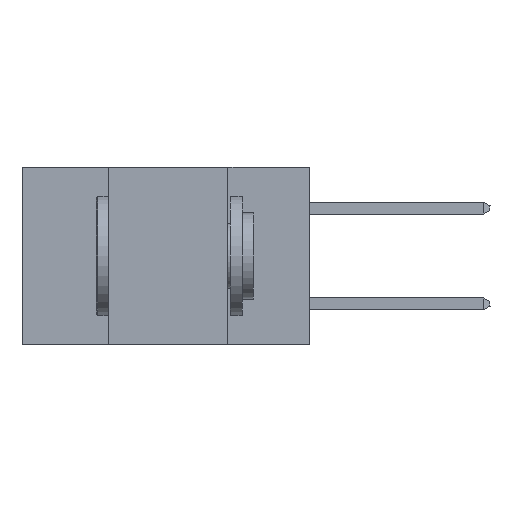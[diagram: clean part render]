
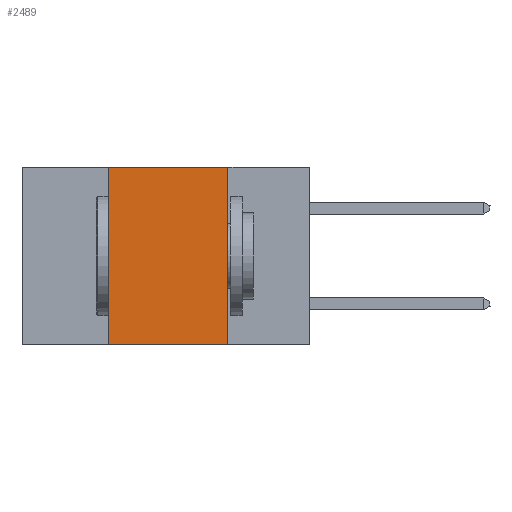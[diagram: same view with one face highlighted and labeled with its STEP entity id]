
A CAD part, left-side view. The second image highlights one B-rep face of the part: STEP entity #2489.
In plain terms, the highlighted planar face has unit normal (-1, 0, 0).
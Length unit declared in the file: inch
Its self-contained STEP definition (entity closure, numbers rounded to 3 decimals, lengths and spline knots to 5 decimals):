
#220 = EDGE_CURVE ( 'NONE', #19680, #14935, #5817, .T. ) ;
#1143 = DIRECTION ( 'NONE',  ( 0., -1., 0. ) ) ;
#2178 = ORIENTED_EDGE ( 'NONE', *, *, #21075, .F. ) ;
#2489 = ADVANCED_FACE ( 'NONE', ( #11546 ), #8200, .F. ) ;
#2505 = CARTESIAN_POINT ( 'NONE',  ( 0., 0.6, 0. ) ) ;
#5447 = CARTESIAN_POINT ( 'NONE',  ( 0., 0.17, -0.37 ) ) ;
#5817 = LINE ( 'NONE', #8719, #15392 ) ;
#6042 = CARTESIAN_POINT ( 'NONE',  ( 0., 0.17, 0. ) ) ;
#6804 = EDGE_LOOP ( 'NONE', ( #15259, #20883, #2178, #8246 ) ) ;
#8001 = EDGE_CURVE ( 'NONE', #12782, #14935, #11087, .T. ) ;
#8118 = DIRECTION ( 'NONE',  ( 1., 0., 0. ) ) ;
#8200 = PLANE ( 'NONE',  #21319 ) ;
#8246 = ORIENTED_EDGE ( 'NONE', *, *, #220, .T. ) ;
#8443 = LINE ( 'NONE', #20289, #19473 ) ;
#8719 = CARTESIAN_POINT ( 'NONE',  ( 0., 0.6, -0.37 ) ) ;
#10296 = DIRECTION ( 'NONE',  ( 0., 0., 1. ) ) ;
#11087 = LINE ( 'NONE', #6042, #20639 ) ;
#11336 = CARTESIAN_POINT ( 'NONE',  ( 0., 0.42, -0.37 ) ) ;
#11546 = FACE_OUTER_BOUND ( 'NONE', #6804, .T. ) ;
#11783 = CARTESIAN_POINT ( 'NONE',  ( 0., 0.42, 0. ) ) ;
#11793 = DIRECTION ( 'NONE',  ( 0., 0., -1. ) ) ;
#11821 = DIRECTION ( 'NONE',  ( 0., 0., -1. ) ) ;
#12782 = VERTEX_POINT ( 'NONE', #19895 ) ;
#13041 = DIRECTION ( 'NONE',  ( 0., -1., 0. ) ) ;
#13751 = LINE ( 'NONE', #16105, #19305 ) ;
#14935 = VERTEX_POINT ( 'NONE', #5447 ) ;
#15259 = ORIENTED_EDGE ( 'NONE', *, *, #8001, .F. ) ;
#15392 = VECTOR ( 'NONE', #1143, 39.37008 ) ;
#16105 = CARTESIAN_POINT ( 'NONE',  ( 0., 0.42, 0. ) ) ;
#19305 = VECTOR ( 'NONE', #10296, 39.37008 ) ;
#19392 = VERTEX_POINT ( 'NONE', #11783 ) ;
#19473 = VECTOR ( 'NONE', #13041, 39.37008 ) ;
#19680 = VERTEX_POINT ( 'NONE', #11336 ) ;
#19895 = CARTESIAN_POINT ( 'NONE',  ( 0., 0.17, 0. ) ) ;
#20289 = CARTESIAN_POINT ( 'NONE',  ( 0., 0.6, 0. ) ) ;
#20639 = VECTOR ( 'NONE', #11793, 39.37008 ) ;
#20883 = ORIENTED_EDGE ( 'NONE', *, *, #23275, .F. ) ;
#21075 = EDGE_CURVE ( 'NONE', #19680, #19392, #13751, .T. ) ;
#21319 = AXIS2_PLACEMENT_3D ( 'NONE', #2505, #8118, #11821 ) ;
#23275 = EDGE_CURVE ( 'NONE', #19392, #12782, #8443, .T. ) ;
